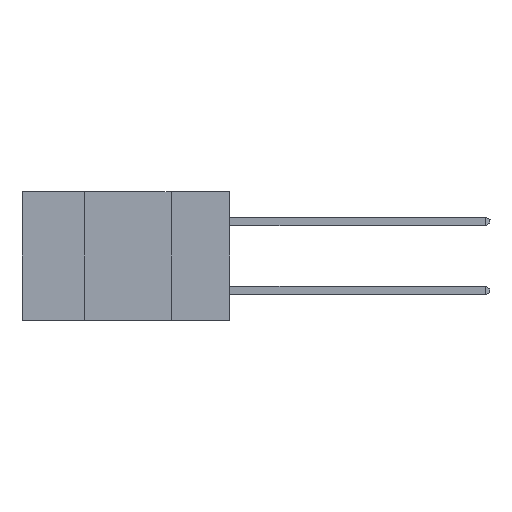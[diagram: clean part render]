
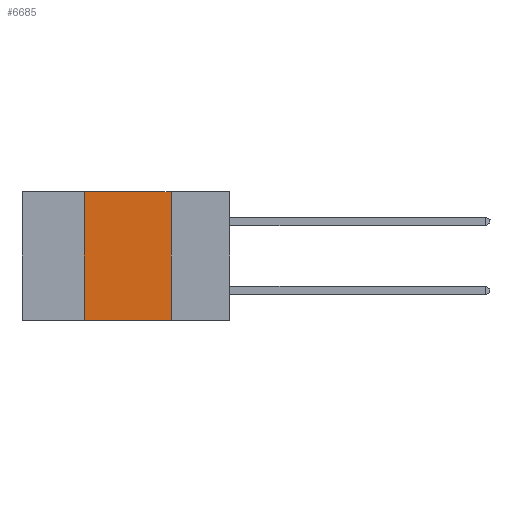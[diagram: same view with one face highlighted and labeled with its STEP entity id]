
A CAD part, left-side view. The second image highlights one B-rep face of the part: STEP entity #6685.
In plain terms, the highlighted planar face has unit normal (-1, 0, 0).
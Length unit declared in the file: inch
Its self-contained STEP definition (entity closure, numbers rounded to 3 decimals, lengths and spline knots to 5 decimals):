
#102 = EDGE_CURVE ( 'NONE', #14043, #6281, #8624, .T. ) ;
#190 = CARTESIAN_POINT ( 'NONE',  ( 0., 0.17, 0. ) ) ;
#623 = DIRECTION ( 'NONE',  ( 0., 0., 1. ) ) ;
#761 = ORIENTED_EDGE ( 'NONE', *, *, #19601, .F. ) ;
#5088 = ORIENTED_EDGE ( 'NONE', *, *, #102, .T. ) ;
#6281 = VERTEX_POINT ( 'NONE', #22119 ) ;
#6393 = CARTESIAN_POINT ( 'NONE',  ( 0., 0.42, 0. ) ) ;
#6431 = EDGE_CURVE ( 'NONE', #11145, #6281, #16323, .T. ) ;
#6685 = ADVANCED_FACE ( 'NONE', ( #16040 ), #12870, .F. ) ;
#7157 = LINE ( 'NONE', #6393, #13047 ) ;
#7792 = ORIENTED_EDGE ( 'NONE', *, *, #12485, .F. ) ;
#8624 = LINE ( 'NONE', #15930, #10309 ) ;
#8821 = DIRECTION ( 'NONE',  ( 1., 0., 0. ) ) ;
#10092 = VERTEX_POINT ( 'NONE', #14132 ) ;
#10309 = VECTOR ( 'NONE', #22807, 39.37008 ) ;
#11145 = VERTEX_POINT ( 'NONE', #190 ) ;
#11584 = CARTESIAN_POINT ( 'NONE',  ( 0., 0.17, 0. ) ) ;
#11934 = DIRECTION ( 'NONE',  ( 0., -1., 0. ) ) ;
#12210 = VECTOR ( 'NONE', #11934, 39.37008 ) ;
#12485 = EDGE_CURVE ( 'NONE', #14043, #10092, #7157, .T. ) ;
#12870 = PLANE ( 'NONE',  #20639 ) ;
#13047 = VECTOR ( 'NONE', #623, 39.37008 ) ;
#14043 = VERTEX_POINT ( 'NONE', #22565 ) ;
#14132 = CARTESIAN_POINT ( 'NONE',  ( 0., 0.42, 0. ) ) ;
#15262 = DIRECTION ( 'NONE',  ( 0., 0., -1. ) ) ;
#15534 = ORIENTED_EDGE ( 'NONE', *, *, #6431, .F. ) ;
#15930 = CARTESIAN_POINT ( 'NONE',  ( 0., 0.6, -0.37 ) ) ;
#16040 = FACE_OUTER_BOUND ( 'NONE', #18735, .T. ) ;
#16323 = LINE ( 'NONE', #11584, #16620 ) ;
#16620 = VECTOR ( 'NONE', #15262, 39.37008 ) ;
#17678 = LINE ( 'NONE', #19006, #12210 ) ;
#18735 = EDGE_LOOP ( 'NONE', ( #15534, #761, #7792, #5088 ) ) ;
#19006 = CARTESIAN_POINT ( 'NONE',  ( 0., 0.6, 0. ) ) ;
#19601 = EDGE_CURVE ( 'NONE', #10092, #11145, #17678, .T. ) ;
#19658 = CARTESIAN_POINT ( 'NONE',  ( 0., 0.6, 0. ) ) ;
#20639 = AXIS2_PLACEMENT_3D ( 'NONE', #19658, #8821, #21478 ) ;
#21478 = DIRECTION ( 'NONE',  ( 0., 0., -1. ) ) ;
#22119 = CARTESIAN_POINT ( 'NONE',  ( 0., 0.17, -0.37 ) ) ;
#22565 = CARTESIAN_POINT ( 'NONE',  ( 0., 0.42, -0.37 ) ) ;
#22807 = DIRECTION ( 'NONE',  ( 0., -1., 0. ) ) ;
